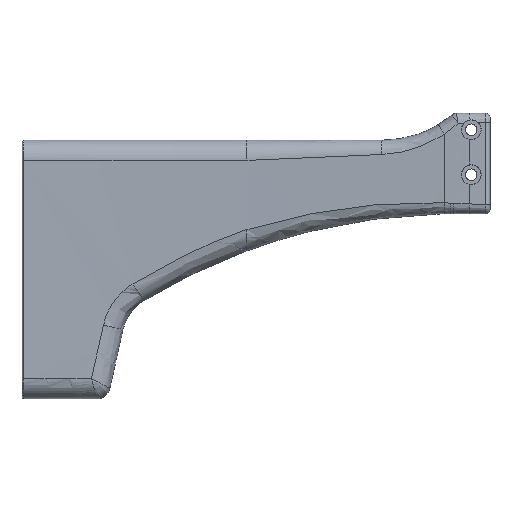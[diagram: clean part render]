
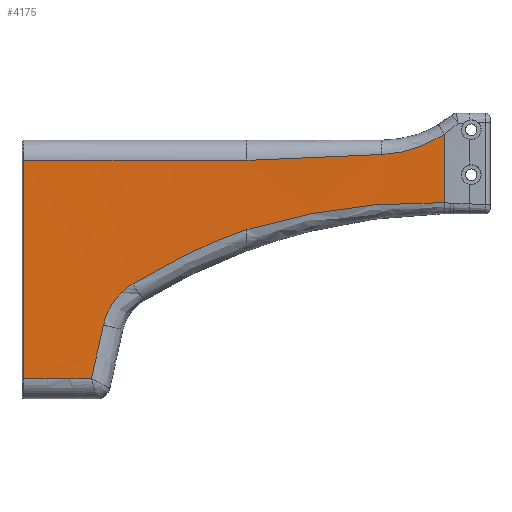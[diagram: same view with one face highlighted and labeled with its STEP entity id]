
A CAD part, left-side view. The second image highlights one B-rep face of the part: STEP entity #4175.
In plain terms, the highlighted cylindrical face has radius 3182.51 mm (diameter 6365.01 mm), a partial arc.
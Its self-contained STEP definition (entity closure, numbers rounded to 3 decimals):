
#177=ELLIPSE('',#4504,14630.042,3182.507);
#295=B_SPLINE_CURVE_WITH_KNOTS('',3,(#8241,#8242,#8243,#8244,#8245),
 .UNSPECIFIED.,.F.,.F.,(4,1,4),(1.162,2.63,3.898),
 .UNSPECIFIED.);
#296=B_SPLINE_CURVE_WITH_KNOTS('',3,(#8246,#8247,#8248,#8249),
 .UNSPECIFIED.,.F.,.F.,(4,4),(0.939,1.162),
 .UNSPECIFIED.);
#300=B_SPLINE_CURVE_WITH_KNOTS('',3,(#8274,#8275,#8276,#8277),
 .UNSPECIFIED.,.F.,.F.,(4,4),(0.329,9.059),
 .UNSPECIFIED.);
#301=B_SPLINE_CURVE_WITH_KNOTS('',3,(#8278,#8279,#8280,#8281),
 .UNSPECIFIED.,.F.,.F.,(4,4),(9.059,9.247),
 .UNSPECIFIED.);
#302=B_SPLINE_CURVE_WITH_KNOTS('',3,(#8283,#8284,#8285,#8286),
 .UNSPECIFIED.,.F.,.F.,(4,4),(3.898,9.923),
 .UNSPECIFIED.);
#303=B_SPLINE_CURVE_WITH_KNOTS('',3,(#8296,#8297,#8298,#8299,#8300),
 .UNSPECIFIED.,.F.,.F.,(4,1,4),(0.,0.999,2.331),
 .UNSPECIFIED.);
#304=B_SPLINE_CURVE_WITH_KNOTS('',3,(#8302,#8303,#8304,#8305),
 .UNSPECIFIED.,.F.,.F.,(4,4),(0.,5.636),
 .UNSPECIFIED.);
#636=FACE_OUTER_BOUND('',#898,.T.);
#898=EDGE_LOOP('',(#3311,#3312,#3313,#3314,#3315,#3316,#3317,#3318,#3319,
#3320,#3321,#3322,#3323));
#1166=LINE('',#8159,#1391);
#1167=LINE('',#8290,#1392);
#1168=LINE('',#8306,#1393);
#1391=VECTOR('',#5145,281.);
#1392=VECTOR('',#5150,10.);
#1393=VECTOR('',#5155,10.);
#1563=CIRCLE('',#4502,3182.507);
#1564=CIRCLE('',#4503,3182.507);
#1840=VERTEX_POINT('',#8153);
#1841=VERTEX_POINT('',#8158);
#1843=VERTEX_POINT('',#8239);
#1844=VERTEX_POINT('',#8240);
#1847=VERTEX_POINT('',#8272);
#1848=VERTEX_POINT('',#8273);
#1849=VERTEX_POINT('',#8282);
#1850=VERTEX_POINT('',#8287);
#1851=VERTEX_POINT('',#8289);
#1852=VERTEX_POINT('',#8291);
#1853=VERTEX_POINT('',#8293);
#1854=VERTEX_POINT('',#8295);
#1855=VERTEX_POINT('',#8301);
#2359=EDGE_CURVE('',#1841,#1840,#1166,.T.);
#2363=EDGE_CURVE('',#1843,#1844,#295,.T.);
#2364=EDGE_CURVE('',#1840,#1843,#296,.T.);
#2368=EDGE_CURVE('',#1847,#1848,#300,.T.);
#2369=EDGE_CURVE('',#1848,#1841,#301,.T.);
#2370=EDGE_CURVE('',#1844,#1849,#302,.T.);
#2371=EDGE_CURVE('',#1849,#1850,#1563,.T.);
#2372=EDGE_CURVE('',#1850,#1851,#1167,.T.);
#2373=EDGE_CURVE('',#1851,#1852,#1564,.T.);
#2374=EDGE_CURVE('',#1852,#1853,#177,.T.);
#2375=EDGE_CURVE('',#1853,#1854,#303,.T.);
#2376=EDGE_CURVE('',#1854,#1855,#304,.T.);
#2377=EDGE_CURVE('',#1855,#1847,#1168,.T.);
#3311=ORIENTED_EDGE('',*,*,#2368,.T.);
#3312=ORIENTED_EDGE('',*,*,#2369,.T.);
#3313=ORIENTED_EDGE('',*,*,#2359,.T.);
#3314=ORIENTED_EDGE('',*,*,#2364,.T.);
#3315=ORIENTED_EDGE('',*,*,#2363,.T.);
#3316=ORIENTED_EDGE('',*,*,#2370,.T.);
#3317=ORIENTED_EDGE('',*,*,#2371,.T.);
#3318=ORIENTED_EDGE('',*,*,#2372,.T.);
#3319=ORIENTED_EDGE('',*,*,#2373,.T.);
#3320=ORIENTED_EDGE('',*,*,#2374,.T.);
#3321=ORIENTED_EDGE('',*,*,#2375,.T.);
#3322=ORIENTED_EDGE('',*,*,#2376,.T.);
#3323=ORIENTED_EDGE('',*,*,#2377,.T.);
#4031=CYLINDRICAL_SURFACE('',#4501,3182.507);
#4175=ADVANCED_FACE('',(#636),#4031,.F.);
#4501=AXIS2_PLACEMENT_3D('',#8271,#5146,#5147);
#4502=AXIS2_PLACEMENT_3D('',#8288,#5148,#5149);
#4503=AXIS2_PLACEMENT_3D('',#8292,#5151,#5152);
#4504=AXIS2_PLACEMENT_3D('',#8294,#5153,#5154);
#5145=DIRECTION('',(0.,0.,1.));
#5146=DIRECTION('center_axis',(0.,0.,1.));
#5147=DIRECTION('ref_axis',(1.,0.021,0.));
#5148=DIRECTION('center_axis',(0.,0.,1.));
#5149=DIRECTION('ref_axis',(1.,0.004,0.));
#5150=DIRECTION('',(0.,0.,-1.));
#5151=DIRECTION('center_axis',(0.,0.,-1.));
#5152=DIRECTION('ref_axis',(1.,0.015,0.));
#5153=DIRECTION('center_axis',(0.,-0.976,
-0.218));
#5154=DIRECTION('ref_axis',(0.,0.218,-0.976));
#5155=DIRECTION('',(0.,0.,-1.));
#8153=CARTESIAN_POINT('',(-1.304,212.319,-257.936));
#8158=CARTESIAN_POINT('',(-1.304,212.319,-288.474));
#8159=CARTESIAN_POINT('',(-1.304,212.319,-248.588));
#8239=CARTESIAN_POINT('',(-1.23,214.194,-259.134));
#8240=CARTESIAN_POINT('',(-0.33,240.019,-266.981));
#8241=CARTESIAN_POINT('Ctrl Pts',(-1.23,214.194,-259.134));
#8242=CARTESIAN_POINT('Ctrl Pts',(-1.068,218.36,-261.676));
#8243=CARTESIAN_POINT('Ctrl Pts',(-0.756,226.772,-265.348));
#8244=CARTESIAN_POINT('Ctrl Pts',(-0.459,235.809,-266.798));
#8245=CARTESIAN_POINT('Ctrl Pts',(-0.33,240.019,-266.981));
#8246=CARTESIAN_POINT('Ctrl Pts',(-1.304,212.319,-257.936));
#8247=CARTESIAN_POINT('Ctrl Pts',(-1.28,212.936,-258.348));
#8248=CARTESIAN_POINT('Ctrl Pts',(-1.255,213.561,-258.748));
#8249=CARTESIAN_POINT('Ctrl Pts',(-1.23,214.194,-259.134));
#8271=CARTESIAN_POINT('Origin',(-3181.326,338.055,-248.588));
#8272=CARTESIAN_POINT('',(0.953,300.,-300.349));
#8273=CARTESIAN_POINT('',(-1.23,214.194,-288.426));
#8274=CARTESIAN_POINT('Ctrl Pts',(0.954,300.001,-300.348));
#8275=CARTESIAN_POINT('Ctrl Pts',(0.625,272.282,-291.823));
#8276=CARTESIAN_POINT('Ctrl Pts',(-0.102,243.19,-287.779));
#8277=CARTESIAN_POINT('Ctrl Pts',(-1.23,214.194,-288.426));
#8278=CARTESIAN_POINT('Ctrl Pts',(-1.23,214.194,-288.426));
#8279=CARTESIAN_POINT('Ctrl Pts',(-1.255,213.569,-288.44));
#8280=CARTESIAN_POINT('Ctrl Pts',(-1.279,212.944,-288.456));
#8281=CARTESIAN_POINT('Ctrl Pts',(-1.304,212.319,-288.474));
#8282=CARTESIAN_POINT('',(0.953,300.,-269.588));
#8283=CARTESIAN_POINT('Ctrl Pts',(-0.33,240.019,-266.981));
#8284=CARTESIAN_POINT('Ctrl Pts',(0.287,260.02,-267.85));
#8285=CARTESIAN_POINT('Ctrl Pts',(0.714,280.007,-268.719));
#8286=CARTESIAN_POINT('Ctrl Pts',(0.953,300.,-269.588));
#8287=CARTESIAN_POINT('',(0.589,399.4,-269.588));
#8288=CARTESIAN_POINT('Origin',(-3181.326,338.055,-269.588));
#8289=CARTESIAN_POINT('',(0.589,399.4,-366.588));
#8290=CARTESIAN_POINT('',(0.589,399.4,-248.588));
#8291=CARTESIAN_POINT('',(1.029,369.123,-366.588));
#8292=CARTESIAN_POINT('Origin',(-3181.326,338.055,-366.588));
#8293=CARTESIAN_POINT('',(1.076,363.826,-342.825));
#8294=CARTESIAN_POINT('Origin',(-3181.326,338.055,-227.191));
#8295=CARTESIAN_POINT('',(1.156,350.652,-324.385));
#8296=CARTESIAN_POINT('Ctrl Pts',(1.076,363.826,-342.825));
#8297=CARTESIAN_POINT('Ctrl Pts',(1.082,363.102,-339.575));
#8298=CARTESIAN_POINT('Ctrl Pts',(1.106,360.099,-332.286));
#8299=CARTESIAN_POINT('Ctrl Pts',(1.141,354.432,-326.695));
#8300=CARTESIAN_POINT('Ctrl Pts',(1.156,350.652,-324.385));
#8301=CARTESIAN_POINT('',(0.953,300.,-300.194));
#8302=CARTESIAN_POINT('Ctrl Pts',(1.156,350.652,-324.385));
#8303=CARTESIAN_POINT('Ctrl Pts',(1.219,334.654,-314.61));
#8304=CARTESIAN_POINT('Ctrl Pts',(1.164,317.65,-306.489));
#8305=CARTESIAN_POINT('Ctrl Pts',(0.953,300.,-300.194));
#8306=CARTESIAN_POINT('',(0.953,300.,-248.588));
